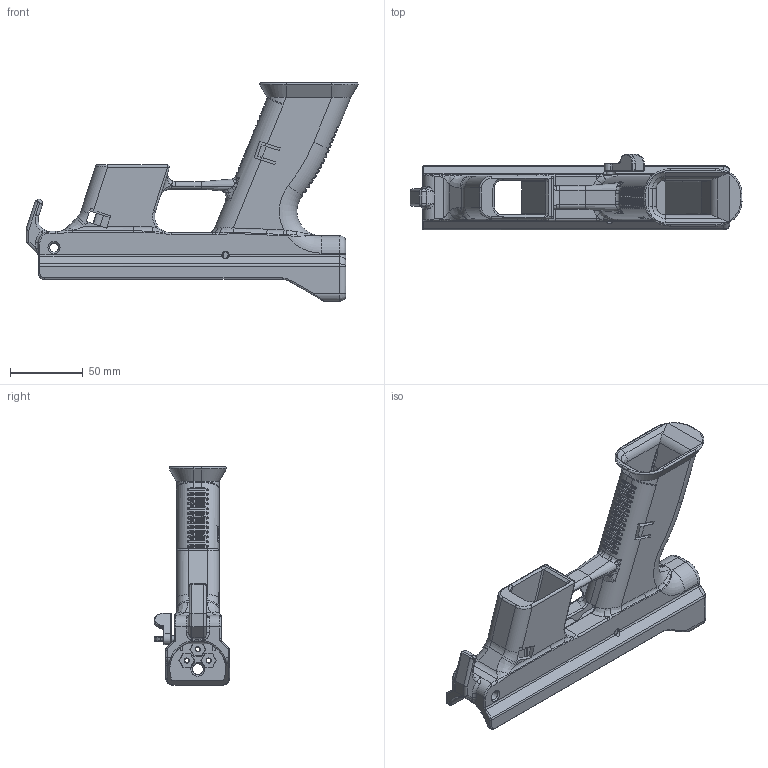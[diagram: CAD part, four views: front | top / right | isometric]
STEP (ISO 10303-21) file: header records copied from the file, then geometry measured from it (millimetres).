
FILE_DESCRIPTION(/* description */ (''),/* implementation_level */ '2;1');
FILE_NAME(/* name */ 'KAP-9 Assembly.step',/* time_stamp */ '2021-07-29T03:03:06-04:00',/* author */ (''),/* organization */ (''),/* preprocessor_version */ 'ST-DEVELOPER v18.1',/* originating_system */ 'Autodesk Translation Framework v10.9.0.1377',/* authorisation */ '');
FILE_SCHEMA (('AUTOMOTIVE_DESIGN { 1 0 10303 214 3 1 1 }'));
Products named in the file (7): KAP-9; KAP-9 Frame; Kimel AP-9 Trigger Group; Trigger Pin; Ejector and Striker Sear Spring Pin; Safety Selector; Safety Selector (1)
Assembly tree (6 placements, depth 3):
  KAP-9
    KAP-9 Frame
    Kimel AP-9 Trigger Group
      Trigger Pin
      Ejector and Striker Sear Spring Pin
      Safety Selector
      Safety Selector (1)
Bounding box: 227.94 x 51.9 x 149.96 mm (x, y, z)
Volume: 250125.4 mm3; surface area: 96654.4 mm2
Topology: 10 solids, 10 shells, 1094 faces, 2899 edges, 1790 vertices
Faces by surface type: plane 346, bspline 343, cylinder 304, torus 78, cone 17, sphere 6
Full cylindrical faces by diameter (mm): 3 x3, 3.9 x1, 4.35 x2, 4.65 x4, 5 x4, 6.3 x5, 7.5 x1
Entity records: 53266 total; most frequent: CARTESIAN_POINT 27721, ORIENTED_EDGE 5746, DIRECTION 4733, EDGE_CURVE 2873, AXIS2_PLACEMENT_3D 1818, VERTEX_POINT 1790, EDGE_LOOP 1131, LINE 1097
